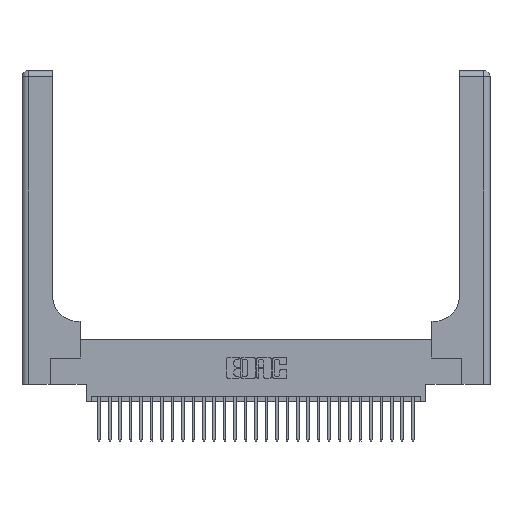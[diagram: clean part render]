
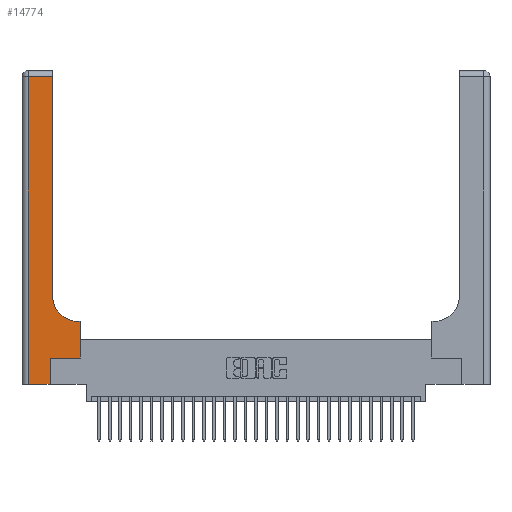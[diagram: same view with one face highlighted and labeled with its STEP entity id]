
A CAD part, top view. The second image highlights one B-rep face of the part: STEP entity #14774.
In plain terms, the highlighted planar face has unit normal (0, 0, 1).
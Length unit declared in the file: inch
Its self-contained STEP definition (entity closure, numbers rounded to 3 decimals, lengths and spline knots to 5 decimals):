
#109 = DIRECTION ( 'NONE',  ( -1., 0., 0. ) ) ;
#200 = CARTESIAN_POINT ( 'NONE',  ( 0.06, 2.94, 0.37 ) ) ;
#510 = VECTOR ( 'NONE', #30536, 39.37008 ) ;
#886 = ORIENTED_EDGE ( 'NONE', *, *, #16662, .T. ) ;
#890 = DIRECTION ( 'NONE',  ( -1., 0., 0. ) ) ;
#1310 = ORIENTED_EDGE ( 'NONE', *, *, #27274, .T. ) ;
#2326 = CARTESIAN_POINT ( 'NONE',  ( 0.2915, 2.94, 0.37 ) ) ;
#2527 = EDGE_CURVE ( 'NONE', #25689, #3683, #22499, .T. ) ;
#2777 = ORIENTED_EDGE ( 'NONE', *, *, #14236, .T. ) ;
#3149 = FACE_OUTER_BOUND ( 'NONE', #26454, .T. ) ;
#3250 = VERTEX_POINT ( 'NONE', #3733 ) ;
#3343 = CARTESIAN_POINT ( 'NONE',  ( 0., 2.94, 0.37 ) ) ;
#3683 = VERTEX_POINT ( 'NONE', #200 ) ;
#3733 = CARTESIAN_POINT ( 'NONE',  ( 0.06, 0., 0.37 ) ) ;
#3740 = DIRECTION ( 'NONE',  ( 0., 0., -1. ) ) ;
#3936 = CARTESIAN_POINT ( 'NONE',  ( 0.5585, 0.25, 0.37 ) ) ;
#4984 = VERTEX_POINT ( 'NONE', #17735 ) ;
#5327 = AXIS2_PLACEMENT_3D ( 'NONE', #23019, #3740, #27789 ) ;
#5891 = VECTOR ( 'NONE', #19675, 39.37008 ) ;
#6152 = DIRECTION ( 'NONE',  ( 0., 1., 0. ) ) ;
#6301 = CARTESIAN_POINT ( 'NONE',  ( 0.5415, 0.6, 0.37 ) ) ;
#6657 = LINE ( 'NONE', #29305, #5891 ) ;
#6716 = CARTESIAN_POINT ( 'NONE',  ( 0.5585, 0.25, 0.37 ) ) ;
#7011 = ORIENTED_EDGE ( 'NONE', *, *, #17325, .T. ) ;
#8296 = LINE ( 'NONE', #8582, #20354 ) ;
#8551 = CARTESIAN_POINT ( 'NONE',  ( 0.5585, 0.6, 0.37 ) ) ;
#8582 = CARTESIAN_POINT ( 'NONE',  ( 0.269, 0.25, 0.37 ) ) ;
#8784 = VERTEX_POINT ( 'NONE', #3936 ) ;
#8941 = VECTOR ( 'NONE', #890, 39.37008 ) ;
#9454 = VECTOR ( 'NONE', #6152, 39.37008 ) ;
#10226 = CARTESIAN_POINT ( 'NONE',  ( 0.5415, 0.85, 0.37 ) ) ;
#10902 = VERTEX_POINT ( 'NONE', #22645 ) ;
#10967 = CARTESIAN_POINT ( 'NONE',  ( 0.06, 3., 0.37 ) ) ;
#10996 = DIRECTION ( 'NONE',  ( 1., 0., 0. ) ) ;
#12586 = LINE ( 'NONE', #23356, #510 ) ;
#12637 = DIRECTION ( 'NONE',  ( 1., 0., 0. ) ) ;
#14236 = EDGE_CURVE ( 'NONE', #4984, #25689, #12586, .T. ) ;
#14774 = ADVANCED_FACE ( 'NONE', ( #3149 ), #25386, .F. ) ;
#15098 = LINE ( 'NONE', #20597, #9454 ) ;
#15101 = AXIS2_PLACEMENT_3D ( 'NONE', #10226, #27031, #12637 ) ;
#16662 = EDGE_CURVE ( 'NONE', #18798, #10902, #15098, .T. ) ;
#16729 = ORIENTED_EDGE ( 'NONE', *, *, #27752, .T. ) ;
#16923 = VECTOR ( 'NONE', #109, 39.37008 ) ;
#16956 = EDGE_CURVE ( 'NONE', #10902, #8784, #8296, .T. ) ;
#17325 = EDGE_CURVE ( 'NONE', #27268, #25081, #30423, .T. ) ;
#17735 = CARTESIAN_POINT ( 'NONE',  ( 0.2915, 0.85, 0.37 ) ) ;
#17969 = ORIENTED_EDGE ( 'NONE', *, *, #20877, .T. ) ;
#18798 = VERTEX_POINT ( 'NONE', #25084 ) ;
#19675 = DIRECTION ( 'NONE',  ( 1., 0., 0. ) ) ;
#20354 = VECTOR ( 'NONE', #10996, 39.37008 ) ;
#20597 = CARTESIAN_POINT ( 'NONE',  ( 0.269, 0., 0.37 ) ) ;
#20877 = EDGE_CURVE ( 'NONE', #25081, #4984, #21412, .T. ) ;
#21412 = CIRCLE ( 'NONE', #15101, 0.25 ) ;
#21709 = EDGE_CURVE ( 'NONE', #8784, #27268, #31128, .T. ) ;
#22499 = LINE ( 'NONE', #3343, #8941 ) ;
#22645 = CARTESIAN_POINT ( 'NONE',  ( 0.269, 0.25, 0.37 ) ) ;
#23019 = CARTESIAN_POINT ( 'NONE',  ( 0., 3., 0.37 ) ) ;
#23356 = CARTESIAN_POINT ( 'NONE',  ( 0.2915, 3., 0.37 ) ) ;
#24233 = CARTESIAN_POINT ( 'NONE',  ( 0.2915, 0.6, 0.37 ) ) ;
#24375 = VECTOR ( 'NONE', #30157, 39.37008 ) ;
#25081 = VERTEX_POINT ( 'NONE', #6301 ) ;
#25084 = CARTESIAN_POINT ( 'NONE',  ( 0.269, 0., 0.37 ) ) ;
#25120 = LINE ( 'NONE', #10967, #24375 ) ;
#25386 = PLANE ( 'NONE',  #5327 ) ;
#25509 = VECTOR ( 'NONE', #30646, 39.37008 ) ;
#25689 = VERTEX_POINT ( 'NONE', #2326 ) ;
#25787 = ORIENTED_EDGE ( 'NONE', *, *, #21709, .T. ) ;
#26454 = EDGE_LOOP ( 'NONE', ( #2777, #30391, #1310, #16729, #886, #26748, #25787, #7011, #17969 ) ) ;
#26748 = ORIENTED_EDGE ( 'NONE', *, *, #16956, .T. ) ;
#27031 = DIRECTION ( 'NONE',  ( 0., 0., -1. ) ) ;
#27268 = VERTEX_POINT ( 'NONE', #8551 ) ;
#27274 = EDGE_CURVE ( 'NONE', #3683, #3250, #25120, .T. ) ;
#27752 = EDGE_CURVE ( 'NONE', #3250, #18798, #6657, .T. ) ;
#27789 = DIRECTION ( 'NONE',  ( -1., 0., 0. ) ) ;
#29305 = CARTESIAN_POINT ( 'NONE',  ( 0., 0., 0.37 ) ) ;
#30157 = DIRECTION ( 'NONE',  ( 0., -1., 0. ) ) ;
#30391 = ORIENTED_EDGE ( 'NONE', *, *, #2527, .T. ) ;
#30423 = LINE ( 'NONE', #24233, #16923 ) ;
#30536 = DIRECTION ( 'NONE',  ( 0., 1., 0. ) ) ;
#30646 = DIRECTION ( 'NONE',  ( 0., 1., 0. ) ) ;
#31128 = LINE ( 'NONE', #6716, #25509 ) ;
